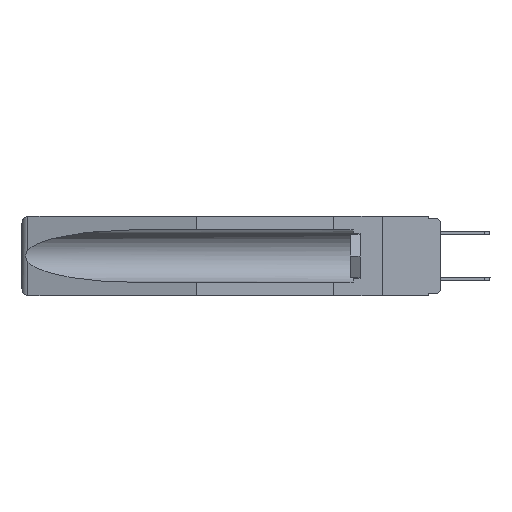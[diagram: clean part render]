
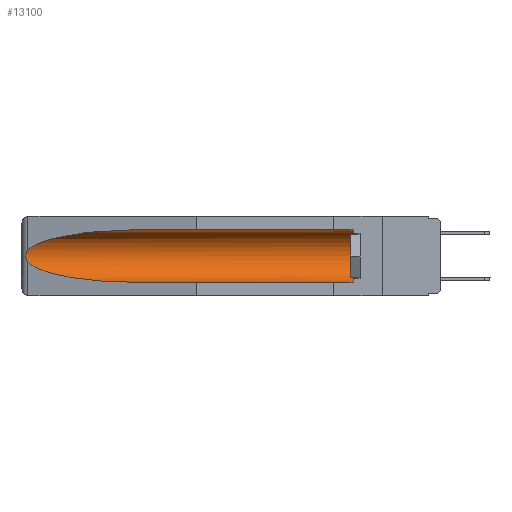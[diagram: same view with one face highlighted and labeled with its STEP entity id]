
A CAD part, left-side view. The second image highlights one B-rep face of the part: STEP entity #13100.
In plain terms, the highlighted cylindrical face has radius 2.857 mm (diameter 5.715 mm), a partial arc.
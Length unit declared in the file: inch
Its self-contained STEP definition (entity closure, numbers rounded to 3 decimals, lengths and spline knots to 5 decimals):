
#93 = VERTEX_POINT ( 'NONE', #19048 ) ;
#1294 = EDGE_CURVE ( 'NONE', #22255, #25128, #11325, .T. ) ;
#2101 = EDGE_CURVE ( 'NONE', #25128, #18404, #20854, .T. ) ;
#3390 = CARTESIAN_POINT ( 'NONE',  ( 0.26537, 1.52718, -0.19328 ) ) ;
#4265 = VECTOR ( 'NONE', #22372, 39.37008 ) ;
#4412 = CARTESIAN_POINT ( 'NONE',  ( 0.155, -0.30754, -0.1715 ) ) ;
#5063 = CARTESIAN_POINT ( 'NONE',  ( 0.155, 0.126, -0.059 ) ) ;
#5372 = VERTEX_POINT ( 'NONE', #23958 ) ;
#5384 = EDGE_CURVE ( 'NONE', #18404, #93, #21353, .T. ) ;
#5456 = CARTESIAN_POINT ( 'NONE',  ( 0.2675, 1.53308, -0.17534 ) ) ;
#5458 = CARTESIAN_POINT ( 'NONE',  ( 0.26537, 1.52718, -0.19328 ) ) ;
#5609 = CARTESIAN_POINT ( 'NONE',  ( 0.25451, 1.48313, -0.09465 ) ) ;
#6895 = CARTESIAN_POINT ( 'NONE',  ( 0.155, 0.126, -0.1715 ) ) ;
#7827 = VECTOR ( 'NONE', #27454, 39.37008 ) ;
#8878 = ORIENTED_EDGE ( 'NONE', *, *, #23782, .T. ) ;
#9764 = CARTESIAN_POINT ( 'NONE',  ( 0.2675, 1.53308, -0.16763 ) ) ;
#10199 = AXIS2_PLACEMENT_3D ( 'NONE', #4412, #25546, #10802 ) ;
#10525 = FACE_OUTER_BOUND ( 'NONE', #14551, .T. ) ;
#10802 = DIRECTION ( 'NONE',  ( 0., 0., 1. ) ) ;
#11301 = CARTESIAN_POINT ( 'NONE',  ( 0.26654, 1.53092, -0.15636 ) ) ;
#11325 = CIRCLE ( 'NONE', #17491, 0.1125 ) ;
#11571 = CARTESIAN_POINT ( 'NONE',  ( 0.26597, 1.52961, -0.15275 ) ) ;
#11615 = ORIENTED_EDGE ( 'NONE', *, *, #21285, .F. ) ;
#13100 = ADVANCED_FACE ( 'NONE', ( #10525 ), #27391, .F. ) ;
#13382 = CARTESIAN_POINT ( 'NONE',  ( 0.26597, 1.5296, -0.19026 ) ) ;
#14188 = LINE ( 'NONE', #22691, #4265 ) ;
#14551 = EDGE_LOOP ( 'NONE', ( #17205, #19355, #8878, #11615, #23920, #21877 ) ) ;
#16403 = CARTESIAN_POINT ( 'NONE',  ( 0.26537, 1.52718, -0.14972 ) ) ;
#16677 = CARTESIAN_POINT ( 'NONE',  ( 0.155, -0.30754, -0.059 ) ) ;
#17205 = ORIENTED_EDGE ( 'NONE', *, *, #5384, .T. ) ;
#17491 = AXIS2_PLACEMENT_3D ( 'NONE', #6895, #25798, #26087 ) ;
#17942 = CARTESIAN_POINT ( 'NONE',  ( 0.26537, 1.52718, -0.14972 ) ) ;
#18082 = CARTESIAN_POINT ( 'NONE',  ( 0.2673, 1.53269, -0.17917 ) ) ;
#18404 = VERTEX_POINT ( 'NONE', #18460 ) ;
#18460 = CARTESIAN_POINT ( 'NONE',  ( 0.155, 1.07973, -0.059 ) ) ;
#19048 = CARTESIAN_POINT ( 'NONE',  ( 0.26537, 1.52718, -0.14972 ) ) ;
#19355 = ORIENTED_EDGE ( 'NONE', *, *, #21116, .T. ) ;
#19432 = CARTESIAN_POINT ( 'NONE',  ( 0.155, 0.126, -0.284 ) ) ;
#20019 = CARTESIAN_POINT ( 'NONE',  ( 0.21114, 1.30732, -0.284 ) ) ;
#20123 =( BOUNDED_CURVE ( )  B_SPLINE_CURVE ( 3, ( #5458, #24496, #20019, #22693 ),
 .UNSPECIFIED., .F., .T. ) 
 B_SPLINE_CURVE_WITH_KNOTS ( ( 4, 4 ),
 ( 0.1948, 1.5708 ),
 .UNSPECIFIED. ) 
 CURVE ( )  GEOMETRIC_REPRESENTATION_ITEM ( )  RATIONAL_B_SPLINE_CURVE ( ( 1., 0.848, 0.848, 1. ) ) 
 REPRESENTATION_ITEM ( '' )  );
#20308 = CARTESIAN_POINT ( 'NONE',  ( 0.21114, 1.30732, -0.059 ) ) ;
#20854 = LINE ( 'NONE', #16677, #7827 ) ;
#21116 = EDGE_CURVE ( 'NONE', #93, #5372, #25430, .T. ) ;
#21285 = EDGE_CURVE ( 'NONE', #22255, #24452, #14188, .T. ) ;
#21353 =( BOUNDED_CURVE ( )  B_SPLINE_CURVE ( 3, ( #24503, #20308, #5609, #16403 ),
 .UNSPECIFIED., .F., .T. ) 
 B_SPLINE_CURVE_WITH_KNOTS ( ( 4, 4 ),
 ( 4.71239, 6.08839 ),
 .UNSPECIFIED. ) 
 CURVE ( )  GEOMETRIC_REPRESENTATION_ITEM ( )  RATIONAL_B_SPLINE_CURVE ( ( 1., 0.848, 0.848, 1. ) ) 
 REPRESENTATION_ITEM ( '' )  );
#21857 = CARTESIAN_POINT ( 'NONE',  ( 0.26655, 1.53094, -0.18657 ) ) ;
#21877 = ORIENTED_EDGE ( 'NONE', *, *, #2101, .T. ) ;
#22255 = VERTEX_POINT ( 'NONE', #19432 ) ;
#22372 = DIRECTION ( 'NONE',  ( 0., 1., 0. ) ) ;
#22691 = CARTESIAN_POINT ( 'NONE',  ( 0.155, -0.30754, -0.284 ) ) ;
#22693 = CARTESIAN_POINT ( 'NONE',  ( 0.155, 1.07973, -0.284 ) ) ;
#23310 = CARTESIAN_POINT ( 'NONE',  ( 0.155, 1.07973, -0.284 ) ) ;
#23782 = EDGE_CURVE ( 'NONE', #5372, #24452, #20123, .T. ) ;
#23920 = ORIENTED_EDGE ( 'NONE', *, *, #1294, .T. ) ;
#23958 = CARTESIAN_POINT ( 'NONE',  ( 0.26537, 1.52718, -0.19328 ) ) ;
#24083 = CARTESIAN_POINT ( 'NONE',  ( 0.2673, 1.5327, -0.16383 ) ) ;
#24452 = VERTEX_POINT ( 'NONE', #23310 ) ;
#24496 = CARTESIAN_POINT ( 'NONE',  ( 0.25451, 1.48313, -0.24835 ) ) ;
#24503 = CARTESIAN_POINT ( 'NONE',  ( 0.155, 1.07973, -0.059 ) ) ;
#25128 = VERTEX_POINT ( 'NONE', #5063 ) ;
#25430 = B_SPLINE_CURVE_WITH_KNOTS ( 'NONE', 3,
 ( #17942, #11571, #11301, #24083, #9764, #5456, #18082, #21857, #13382, #3390 ),
 .UNSPECIFIED., .F., .F.,
 ( 4, 2, 2, 2, 4 ),
 ( 0., 0.00029, 0.00058, 0.00087, 0.00117 ),
 .UNSPECIFIED. ) ;
#25546 = DIRECTION ( 'NONE',  ( 0., 1., 0. ) ) ;
#25798 = DIRECTION ( 'NONE',  ( 0., -1., 0. ) ) ;
#26087 = DIRECTION ( 'NONE',  ( 0., 0., 1. ) ) ;
#27391 = CYLINDRICAL_SURFACE ( 'NONE', #10199, 0.1125 ) ;
#27454 = DIRECTION ( 'NONE',  ( 0., 1., 0. ) ) ;
